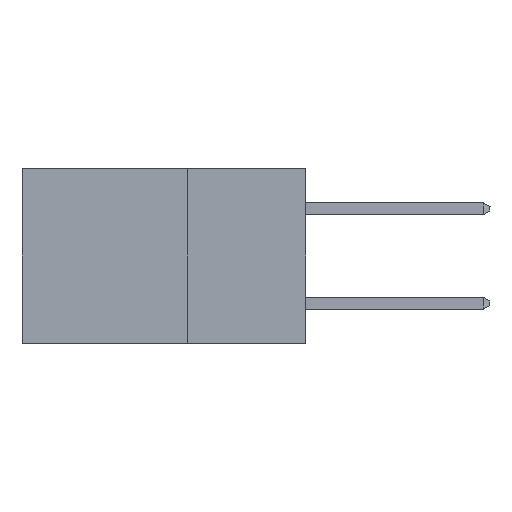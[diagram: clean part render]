
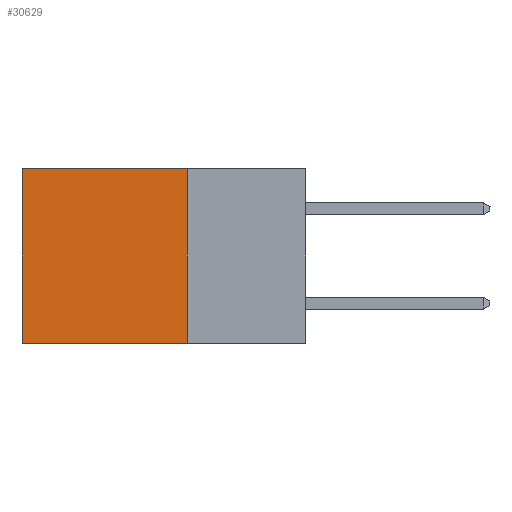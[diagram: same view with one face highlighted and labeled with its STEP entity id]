
A CAD part, left-side view. The second image highlights one B-rep face of the part: STEP entity #30629.
In plain terms, the highlighted planar face has unit normal (-1, 0, 0).
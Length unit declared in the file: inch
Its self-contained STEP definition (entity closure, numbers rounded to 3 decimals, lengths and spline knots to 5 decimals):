
#359 = CARTESIAN_POINT ( 'NONE',  ( 0.298, 0.6, -0.37 ) ) ;
#962 = CARTESIAN_POINT ( 'NONE',  ( 0.298, 0.6, 0. ) ) ;
#2453 = LINE ( 'NONE', #7788, #26306 ) ;
#3033 = FACE_OUTER_BOUND ( 'NONE', #4589, .T. ) ;
#3363 = ORIENTED_EDGE ( 'NONE', *, *, #11223, .T. ) ;
#3879 = DIRECTION ( 'NONE',  ( 1., 0., 0. ) ) ;
#4589 = EDGE_LOOP ( 'NONE', ( #11003, #9231, #11009, #3363 ) ) ;
#5182 = VERTEX_POINT ( 'NONE', #26747 ) ;
#6986 = EDGE_CURVE ( 'NONE', #5182, #28277, #2453, .T. ) ;
#7788 = CARTESIAN_POINT ( 'NONE',  ( 0.298, 0.25, -0.37 ) ) ;
#7845 = VERTEX_POINT ( 'NONE', #27631 ) ;
#9231 = ORIENTED_EDGE ( 'NONE', *, *, #6986, .F. ) ;
#11003 = ORIENTED_EDGE ( 'NONE', *, *, #23744, .T. ) ;
#11009 = ORIENTED_EDGE ( 'NONE', *, *, #23921, .F. ) ;
#11223 = EDGE_CURVE ( 'NONE', #7845, #29791, #14709, .T. ) ;
#11346 = PLANE ( 'NONE',  #24184 ) ;
#13918 = CARTESIAN_POINT ( 'NONE',  ( 0.298, 0.6, 0. ) ) ;
#14200 = LINE ( 'NONE', #13918, #27842 ) ;
#14709 = LINE ( 'NONE', #21469, #26837 ) ;
#20004 = DIRECTION ( 'NONE',  ( 0., 1., 0. ) ) ;
#21133 = DIRECTION ( 'NONE',  ( 0., 0., -1. ) ) ;
#21469 = CARTESIAN_POINT ( 'NONE',  ( 0.298, 0.25, 0. ) ) ;
#21795 = DIRECTION ( 'NONE',  ( 0., 0., -1. ) ) ;
#21809 = VECTOR ( 'NONE', #21795, 39.37008 ) ;
#23744 = EDGE_CURVE ( 'NONE', #29791, #28277, #14200, .T. ) ;
#23890 = DIRECTION ( 'NONE',  ( 0., 1., 0. ) ) ;
#23921 = EDGE_CURVE ( 'NONE', #7845, #5182, #28947, .T. ) ;
#24184 = AXIS2_PLACEMENT_3D ( 'NONE', #25854, #3879, #21133 ) ;
#25854 = CARTESIAN_POINT ( 'NONE',  ( 0.298, 0.25, 0. ) ) ;
#26306 = VECTOR ( 'NONE', #20004, 39.37008 ) ;
#26747 = CARTESIAN_POINT ( 'NONE',  ( 0.298, 0.25, -0.37 ) ) ;
#26837 = VECTOR ( 'NONE', #23890, 39.37008 ) ;
#27631 = CARTESIAN_POINT ( 'NONE',  ( 0.298, 0.25, 0. ) ) ;
#27842 = VECTOR ( 'NONE', #30867, 39.37008 ) ;
#28277 = VERTEX_POINT ( 'NONE', #359 ) ;
#28947 = LINE ( 'NONE', #31364, #21809 ) ;
#29791 = VERTEX_POINT ( 'NONE', #962 ) ;
#30629 = ADVANCED_FACE ( 'NONE', ( #3033 ), #11346, .F. ) ;
#30867 = DIRECTION ( 'NONE',  ( 0., 0., -1. ) ) ;
#31364 = CARTESIAN_POINT ( 'NONE',  ( 0.298, 0.25, 0. ) ) ;
